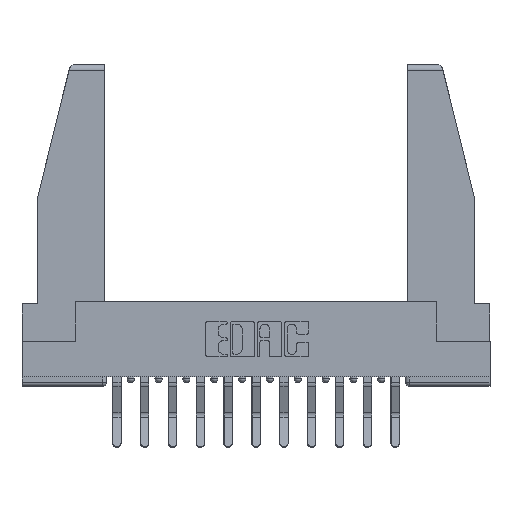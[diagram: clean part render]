
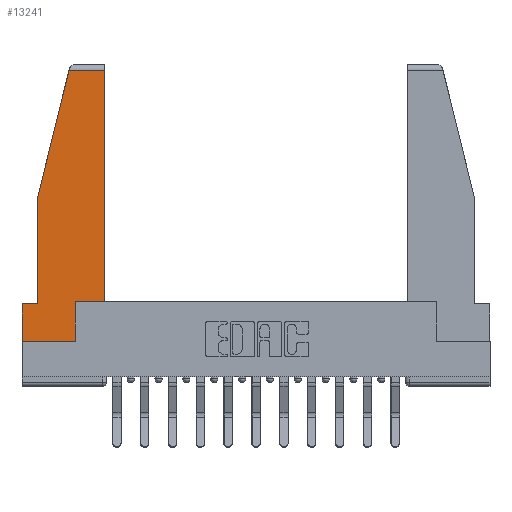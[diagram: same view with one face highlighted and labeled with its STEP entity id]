
A CAD part, top view. The second image highlights one B-rep face of the part: STEP entity #13241.
In plain terms, the highlighted planar face has unit normal (0, 0, 1).
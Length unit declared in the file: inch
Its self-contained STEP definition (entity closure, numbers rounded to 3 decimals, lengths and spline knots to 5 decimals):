
#108 = EDGE_CURVE ( 'NONE', #4622, #8753, #15972, .T. ) ;
#193 = LINE ( 'NONE', #5354, #15621 ) ;
#236 = EDGE_CURVE ( 'NONE', #2468, #4622, #14792, .T. ) ;
#696 = EDGE_CURVE ( 'NONE', #8753, #8531, #9107, .T. ) ;
#865 = VECTOR ( 'NONE', #15083, 39.37008 ) ;
#1970 = CARTESIAN_POINT ( 'NONE',  ( 0.461, 1.52, 0. ) ) ;
#2015 = EDGE_CURVE ( 'NONE', #8531, #11490, #5786, .T. ) ;
#2104 = CARTESIAN_POINT ( 'NONE',  ( 0.461, 0.223, 0. ) ) ;
#2195 = DIRECTION ( 'NONE',  ( 1., 0., 0. ) ) ;
#2318 = CARTESIAN_POINT ( 'NONE',  ( 0., 0.21, 0. ) ) ;
#2468 = VERTEX_POINT ( 'NONE', #1970 ) ;
#3033 = EDGE_CURVE ( 'NONE', #5301, #9777, #13743, .T. ) ;
#3652 = VECTOR ( 'NONE', #4290, 39.37008 ) ;
#4290 = DIRECTION ( 'NONE',  ( -0.239, -0.971, 0. ) ) ;
#4622 = VERTEX_POINT ( 'NONE', #14607 ) ;
#4809 = CARTESIAN_POINT ( 'NONE',  ( 0.461, 0.223, 0. ) ) ;
#4840 = VECTOR ( 'NONE', #6974, 39.37008 ) ;
#4996 = EDGE_CURVE ( 'NONE', #9777, #7263, #193, .T. ) ;
#5301 = VERTEX_POINT ( 'NONE', #9546 ) ;
#5354 = CARTESIAN_POINT ( 'NONE',  ( 0.297, 0., 0. ) ) ;
#5410 = DIRECTION ( 'NONE',  ( 0., 1., 0. ) ) ;
#5463 = EDGE_CURVE ( 'NONE', #11490, #5301, #11683, .T. ) ;
#5668 = CARTESIAN_POINT ( 'NONE',  ( 0., 0.21, 0. ) ) ;
#5786 = LINE ( 'NONE', #2318, #6187 ) ;
#5877 = ORIENTED_EDGE ( 'NONE', *, *, #9470, .T. ) ;
#5908 = ORIENTED_EDGE ( 'NONE', *, *, #14912, .T. ) ;
#5931 = PLANE ( 'NONE',  #11449 ) ;
#6187 = VECTOR ( 'NONE', #8556, 39.37008 ) ;
#6430 = VECTOR ( 'NONE', #7474, 39.37008 ) ;
#6542 = EDGE_LOOP ( 'NONE', ( #5877, #7528, #14152, #10520, #14548, #8216, #8242, #10281, #5908 ) ) ;
#6586 = CARTESIAN_POINT ( 'NONE',  ( 0.297, 0.223, 0. ) ) ;
#6917 = FACE_OUTER_BOUND ( 'NONE', #6542, .T. ) ;
#6974 = DIRECTION ( 'NONE',  ( -1., 0., 0. ) ) ;
#7124 = DIRECTION ( 'NONE',  ( 0., 1., 0. ) ) ;
#7263 = VERTEX_POINT ( 'NONE', #6586 ) ;
#7474 = DIRECTION ( 'NONE',  ( 0., -1., 0. ) ) ;
#7528 = ORIENTED_EDGE ( 'NONE', *, *, #236, .T. ) ;
#7712 = VECTOR ( 'NONE', #15917, 39.37008 ) ;
#8216 = ORIENTED_EDGE ( 'NONE', *, *, #5463, .T. ) ;
#8242 = ORIENTED_EDGE ( 'NONE', *, *, #3033, .T. ) ;
#8299 = LINE ( 'NONE', #10044, #865 ) ;
#8531 = VERTEX_POINT ( 'NONE', #12999 ) ;
#8556 = DIRECTION ( 'NONE',  ( -1., 0., 0. ) ) ;
#8733 = CARTESIAN_POINT ( 'NONE',  ( 0., 0.21, 0. ) ) ;
#8753 = VERTEX_POINT ( 'NONE', #10689 ) ;
#9107 = LINE ( 'NONE', #12828, #14995 ) ;
#9470 = EDGE_CURVE ( 'NONE', #15518, #2468, #13678, .T. ) ;
#9546 = CARTESIAN_POINT ( 'NONE',  ( 0., 0., 0. ) ) ;
#9575 = DIRECTION ( 'NONE',  ( 0., 0., 1. ) ) ;
#9600 = CARTESIAN_POINT ( 'NONE',  ( 0.297, 0., 0. ) ) ;
#9777 = VERTEX_POINT ( 'NONE', #9600 ) ;
#9954 = VECTOR ( 'NONE', #7124, 39.37008 ) ;
#10044 = CARTESIAN_POINT ( 'NONE',  ( 0.297, 0.223, 0. ) ) ;
#10281 = ORIENTED_EDGE ( 'NONE', *, *, #4996, .T. ) ;
#10520 = ORIENTED_EDGE ( 'NONE', *, *, #696, .T. ) ;
#10689 = CARTESIAN_POINT ( 'NONE',  ( 0.086, 0.8, 0. ) ) ;
#11449 = AXIS2_PLACEMENT_3D ( 'NONE', #14653, #9575, #2195 ) ;
#11490 = VERTEX_POINT ( 'NONE', #5668 ) ;
#11683 = LINE ( 'NONE', #8733, #6430 ) ;
#12251 = CARTESIAN_POINT ( 'NONE',  ( 0., 0., 0. ) ) ;
#12721 = DIRECTION ( 'NONE',  ( 0., -1., 0. ) ) ;
#12828 = CARTESIAN_POINT ( 'NONE',  ( 0.086, 0.8, 0. ) ) ;
#12908 = CARTESIAN_POINT ( 'NONE',  ( 0.271, 1.55, 0. ) ) ;
#12999 = CARTESIAN_POINT ( 'NONE',  ( 0.086, 0.21, 0. ) ) ;
#13178 = CARTESIAN_POINT ( 'NONE',  ( 0., 1.52, 0. ) ) ;
#13241 = ADVANCED_FACE ( 'NONE', ( #6917 ), #5931, .T. ) ;
#13678 = LINE ( 'NONE', #2104, #9954 ) ;
#13743 = LINE ( 'NONE', #12251, #7712 ) ;
#14152 = ORIENTED_EDGE ( 'NONE', *, *, #108, .T. ) ;
#14548 = ORIENTED_EDGE ( 'NONE', *, *, #2015, .T. ) ;
#14607 = CARTESIAN_POINT ( 'NONE',  ( 0.2636, 1.52, 0. ) ) ;
#14653 = CARTESIAN_POINT ( 'NONE',  ( 0., 0., 0. ) ) ;
#14792 = LINE ( 'NONE', #13178, #4840 ) ;
#14912 = EDGE_CURVE ( 'NONE', #7263, #15518, #8299, .T. ) ;
#14995 = VECTOR ( 'NONE', #12721, 39.37008 ) ;
#15083 = DIRECTION ( 'NONE',  ( 1., 0., 0. ) ) ;
#15518 = VERTEX_POINT ( 'NONE', #4809 ) ;
#15621 = VECTOR ( 'NONE', #5410, 39.37008 ) ;
#15917 = DIRECTION ( 'NONE',  ( 1., 0., 0. ) ) ;
#15972 = LINE ( 'NONE', #12908, #3652 ) ;
